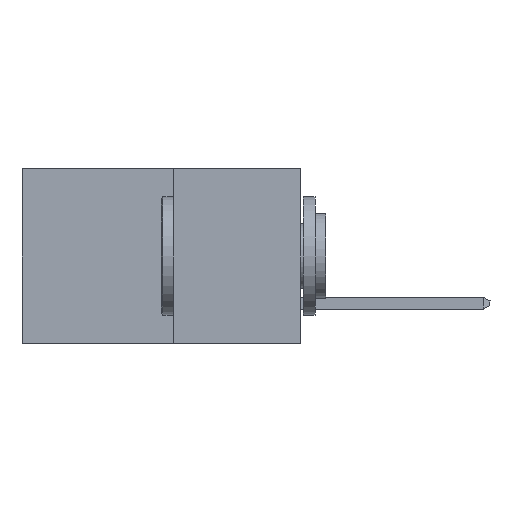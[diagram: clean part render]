
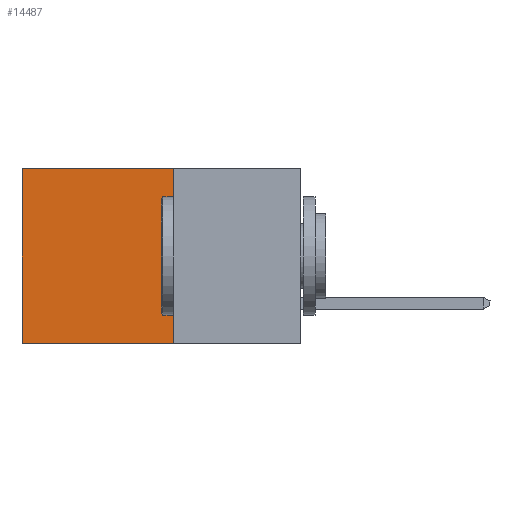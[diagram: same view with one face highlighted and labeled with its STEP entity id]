
A CAD part, left-side view. The second image highlights one B-rep face of the part: STEP entity #14487.
In plain terms, the highlighted planar face has unit normal (-1, 0, 0).
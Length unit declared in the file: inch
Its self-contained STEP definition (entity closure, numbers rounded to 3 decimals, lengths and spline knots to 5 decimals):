
#865 = DIRECTION ( 'NONE',  ( 0., 0., -1. ) ) ;
#1027 = LINE ( 'NONE', #14367, #21204 ) ;
#2326 = DIRECTION ( 'NONE',  ( 0., 0., -1. ) ) ;
#3091 = CARTESIAN_POINT ( 'NONE',  ( 0.277, 0.27, -0.37 ) ) ;
#5137 = EDGE_CURVE ( 'NONE', #30377, #10602, #26057, .T. ) ;
#6119 = ORIENTED_EDGE ( 'NONE', *, *, #5137, .F. ) ;
#6185 = EDGE_LOOP ( 'NONE', ( #8461, #23249, #6119, #7539 ) ) ;
#6254 = VERTEX_POINT ( 'NONE', #33351 ) ;
#6449 = DIRECTION ( 'NONE',  ( 0., 1., 0. ) ) ;
#7539 = ORIENTED_EDGE ( 'NONE', *, *, #21832, .T. ) ;
#8461 = ORIENTED_EDGE ( 'NONE', *, *, #18051, .T. ) ;
#10602 = VERTEX_POINT ( 'NONE', #3091 ) ;
#12362 = VECTOR ( 'NONE', #21103, 39.37008 ) ;
#12802 = CARTESIAN_POINT ( 'NONE',  ( 0.277, 0.27, -0.37 ) ) ;
#14367 = CARTESIAN_POINT ( 'NONE',  ( 0.277, 0.27, 0. ) ) ;
#14487 = ADVANCED_FACE ( 'NONE', ( #18281 ), #30616, .F. ) ;
#15568 = CARTESIAN_POINT ( 'NONE',  ( 0.277, 0.59, -0.37 ) ) ;
#15589 = AXIS2_PLACEMENT_3D ( 'NONE', #30801, #30429, #30388 ) ;
#16436 = LINE ( 'NONE', #15568, #31040 ) ;
#18051 = EDGE_CURVE ( 'NONE', #6254, #18210, #16436, .T. ) ;
#18164 = EDGE_CURVE ( 'NONE', #10602, #18210, #33876, .T. ) ;
#18210 = VERTEX_POINT ( 'NONE', #29027 ) ;
#18281 = FACE_OUTER_BOUND ( 'NONE', #6185, .T. ) ;
#21103 = DIRECTION ( 'NONE',  ( 0., 1., 0. ) ) ;
#21204 = VECTOR ( 'NONE', #6449, 39.37008 ) ;
#21832 = EDGE_CURVE ( 'NONE', #30377, #6254, #1027, .T. ) ;
#23249 = ORIENTED_EDGE ( 'NONE', *, *, #18164, .F. ) ;
#25255 = VECTOR ( 'NONE', #865, 39.37008 ) ;
#26057 = LINE ( 'NONE', #12802, #25255 ) ;
#29027 = CARTESIAN_POINT ( 'NONE',  ( 0.277, 0.59, -0.37 ) ) ;
#30377 = VERTEX_POINT ( 'NONE', #31045 ) ;
#30388 = DIRECTION ( 'NONE',  ( 0., 0., -1. ) ) ;
#30429 = DIRECTION ( 'NONE',  ( 1., 0., 0. ) ) ;
#30616 = PLANE ( 'NONE',  #15589 ) ;
#30801 = CARTESIAN_POINT ( 'NONE',  ( 0.277, 0.27, -0.37 ) ) ;
#31040 = VECTOR ( 'NONE', #2326, 39.37008 ) ;
#31045 = CARTESIAN_POINT ( 'NONE',  ( 0.277, 0.27, 0. ) ) ;
#31425 = CARTESIAN_POINT ( 'NONE',  ( 0.277, 0.27, -0.37 ) ) ;
#33351 = CARTESIAN_POINT ( 'NONE',  ( 0.277, 0.59, 0. ) ) ;
#33876 = LINE ( 'NONE', #31425, #12362 ) ;
